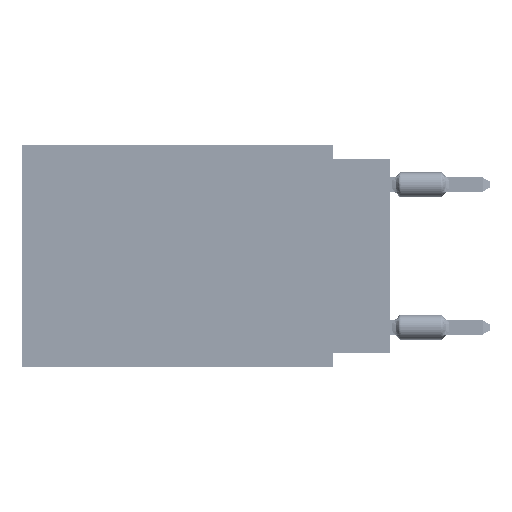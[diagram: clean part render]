
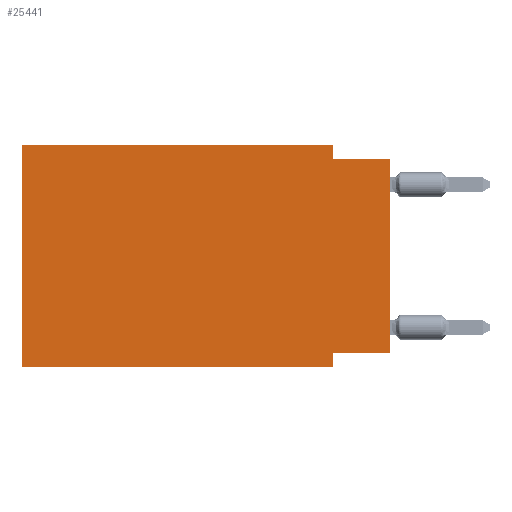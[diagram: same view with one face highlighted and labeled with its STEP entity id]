
A CAD part, left-side view. The second image highlights one B-rep face of the part: STEP entity #25441.
In plain terms, the highlighted planar face has unit normal (-1, 0, 0).
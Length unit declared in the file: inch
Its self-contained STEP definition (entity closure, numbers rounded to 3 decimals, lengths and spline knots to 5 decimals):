
#32 = CARTESIAN_POINT ( 'NONE',  ( 0., 0.645, 0. ) ) ;
#4018 = AXIS2_PLACEMENT_3D ( 'NONE', #32, #38102, #14504 ) ;
#5828 = ORIENTED_EDGE ( 'NONE', *, *, #41558, .F. ) ;
#6323 = EDGE_LOOP ( 'NONE', ( #60148, #13695, #19255, #13734, #5828, #16120, #12547, #10159 ) ) ;
#8177 = CARTESIAN_POINT ( 'NONE',  ( 0., 0.1, -0.39 ) ) ;
#9044 = VECTOR ( 'NONE', #53510, 39.37008 ) ;
#9643 = CARTESIAN_POINT ( 'NONE',  ( 0., 0.645, -0.39 ) ) ;
#9696 = EDGE_CURVE ( 'NONE', #38295, #12204, #55399, .T. ) ;
#9785 = LINE ( 'NONE', #57915, #9044 ) ;
#10159 = ORIENTED_EDGE ( 'NONE', *, *, #14582, .F. ) ;
#11586 = LINE ( 'NONE', #30769, #25911 ) ;
#12204 = VERTEX_POINT ( 'NONE', #36219 ) ;
#12547 = ORIENTED_EDGE ( 'NONE', *, *, #37320, .F. ) ;
#12931 = VECTOR ( 'NONE', #58764, 39.37008 ) ;
#13695 = ORIENTED_EDGE ( 'NONE', *, *, #9696, .F. ) ;
#13734 = ORIENTED_EDGE ( 'NONE', *, *, #28630, .F. ) ;
#13810 = CARTESIAN_POINT ( 'NONE',  ( 0., 0.1, -0.365 ) ) ;
#14504 = DIRECTION ( 'NONE',  ( 0., 0., -1. ) ) ;
#14582 = EDGE_CURVE ( 'NONE', #26860, #50327, #11586, .T. ) ;
#16120 = ORIENTED_EDGE ( 'NONE', *, *, #25432, .T. ) ;
#17201 = DIRECTION ( 'NONE',  ( 0., 0., 1. ) ) ;
#17600 = LINE ( 'NONE', #8177, #31826 ) ;
#19255 = ORIENTED_EDGE ( 'NONE', *, *, #41650, .F. ) ;
#20144 = PLANE ( 'NONE',  #4018 ) ;
#20358 = LINE ( 'NONE', #24779, #12931 ) ;
#21601 = LINE ( 'NONE', #26630, #44785 ) ;
#22159 = CARTESIAN_POINT ( 'NONE',  ( 0., 0.1, 0. ) ) ;
#22635 = DIRECTION ( 'NONE',  ( 0., 0., -1. ) ) ;
#23421 = CARTESIAN_POINT ( 'NONE',  ( 0., 0.1, -0.025 ) ) ;
#24779 = CARTESIAN_POINT ( 'NONE',  ( 0., 0.645, 0. ) ) ;
#25432 = EDGE_CURVE ( 'NONE', #27480, #52846, #9785, .T. ) ;
#25441 = ADVANCED_FACE ( 'NONE', ( #48780 ), #20144, .F. ) ;
#25911 = VECTOR ( 'NONE', #55620, 39.37008 ) ;
#26449 = DIRECTION ( 'NONE',  ( 0., -1., 0. ) ) ;
#26630 = CARTESIAN_POINT ( 'NONE',  ( 0., 0., 0. ) ) ;
#26860 = VERTEX_POINT ( 'NONE', #48564 ) ;
#27480 = VERTEX_POINT ( 'NONE', #9643 ) ;
#28630 = EDGE_CURVE ( 'NONE', #40118, #42141, #36204, .T. ) ;
#30769 = CARTESIAN_POINT ( 'NONE',  ( 0., 0., -0.365 ) ) ;
#31826 = VECTOR ( 'NONE', #22635, 39.37008 ) ;
#36204 = LINE ( 'NONE', #50383, #44877 ) ;
#36219 = CARTESIAN_POINT ( 'NONE',  ( 0., 0., -0.025 ) ) ;
#36696 = CARTESIAN_POINT ( 'NONE',  ( 0., 0.1, 0. ) ) ;
#37320 = EDGE_CURVE ( 'NONE', #50327, #52846, #17600, .T. ) ;
#38102 = DIRECTION ( 'NONE',  ( 1., 0., 0. ) ) ;
#38295 = VERTEX_POINT ( 'NONE', #23421 ) ;
#40118 = VERTEX_POINT ( 'NONE', #41546 ) ;
#41546 = CARTESIAN_POINT ( 'NONE',  ( 0., 0.645, 0. ) ) ;
#41558 = EDGE_CURVE ( 'NONE', #27480, #40118, #20358, .T. ) ;
#41650 = EDGE_CURVE ( 'NONE', #42141, #38295, #56206, .T. ) ;
#42141 = VERTEX_POINT ( 'NONE', #22159 ) ;
#44032 = CARTESIAN_POINT ( 'NONE',  ( 0., 0.1, -0.39 ) ) ;
#44785 = VECTOR ( 'NONE', #17201, 39.37008 ) ;
#44877 = VECTOR ( 'NONE', #50064, 39.37008 ) ;
#48478 = EDGE_CURVE ( 'NONE', #26860, #12204, #21601, .T. ) ;
#48564 = CARTESIAN_POINT ( 'NONE',  ( 0., 0., -0.365 ) ) ;
#48780 = FACE_OUTER_BOUND ( 'NONE', #6323, .T. ) ;
#49740 = CARTESIAN_POINT ( 'NONE',  ( 0., 0., -0.025 ) ) ;
#50064 = DIRECTION ( 'NONE',  ( 0., -1., 0. ) ) ;
#50327 = VERTEX_POINT ( 'NONE', #13810 ) ;
#50383 = CARTESIAN_POINT ( 'NONE',  ( 0., 0.645, 0. ) ) ;
#52846 = VERTEX_POINT ( 'NONE', #44032 ) ;
#53510 = DIRECTION ( 'NONE',  ( 0., -1., 0. ) ) ;
#55399 = LINE ( 'NONE', #49740, #56674 ) ;
#55587 = DIRECTION ( 'NONE',  ( 0., 0., -1. ) ) ;
#55620 = DIRECTION ( 'NONE',  ( 0., 1., 0. ) ) ;
#56206 = LINE ( 'NONE', #36696, #61213 ) ;
#56674 = VECTOR ( 'NONE', #26449, 39.37008 ) ;
#57915 = CARTESIAN_POINT ( 'NONE',  ( 0., 0.645, -0.39 ) ) ;
#58764 = DIRECTION ( 'NONE',  ( 0., 0., 1. ) ) ;
#60148 = ORIENTED_EDGE ( 'NONE', *, *, #48478, .T. ) ;
#61213 = VECTOR ( 'NONE', #55587, 39.37008 ) ;
